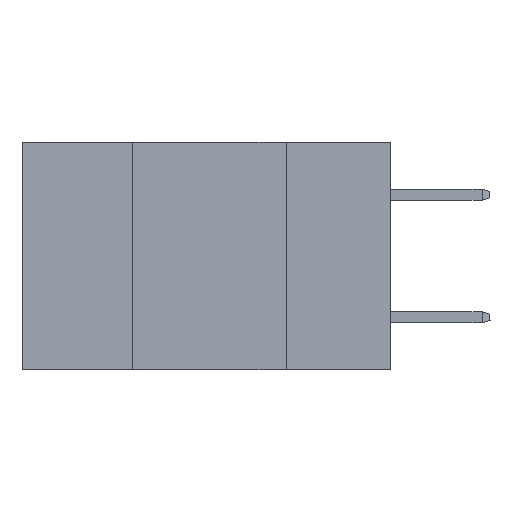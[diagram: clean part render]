
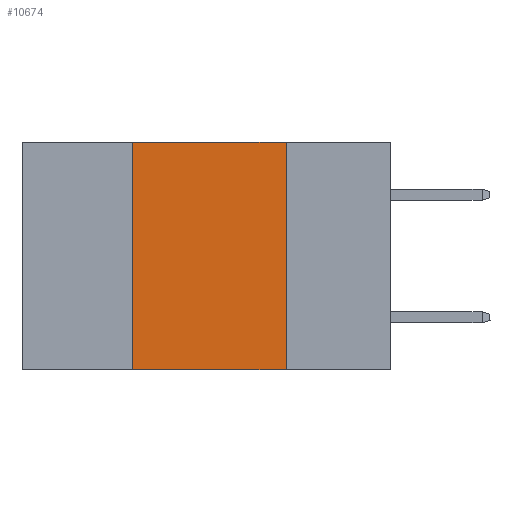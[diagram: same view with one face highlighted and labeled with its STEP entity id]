
A CAD part, left-side view. The second image highlights one B-rep face of the part: STEP entity #10674.
In plain terms, the highlighted planar face has unit normal (-1, 0, 0).
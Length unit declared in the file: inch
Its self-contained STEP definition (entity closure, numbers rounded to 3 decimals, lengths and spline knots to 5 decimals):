
#13 = PLANE ( 'NONE',  #9942 ) ;
#1749 = LINE ( 'NONE', #10028, #11382 ) ;
#1884 = VERTEX_POINT ( 'NONE', #17189 ) ;
#2172 = LINE ( 'NONE', #11243, #21198 ) ;
#3057 = LINE ( 'NONE', #11791, #22034 ) ;
#3492 = EDGE_CURVE ( 'NONE', #21601, #15595, #1749, .T. ) ;
#4226 = CARTESIAN_POINT ( 'NONE',  ( 0., 0.17, 0. ) ) ;
#4954 = VECTOR ( 'NONE', #22202, 39.37008 ) ;
#5994 = DIRECTION ( 'NONE',  ( 1., 0., 0. ) ) ;
#6545 = EDGE_CURVE ( 'NONE', #15595, #11756, #2172, .T. ) ;
#6612 = EDGE_CURVE ( 'NONE', #1884, #21601, #10068, .T. ) ;
#6679 = EDGE_CURVE ( 'NONE', #1884, #11756, #3057, .T. ) ;
#7358 = ORIENTED_EDGE ( 'NONE', *, *, #6545, .F. ) ;
#7449 = ORIENTED_EDGE ( 'NONE', *, *, #3492, .F. ) ;
#7571 = ORIENTED_EDGE ( 'NONE', *, *, #6612, .F. ) ;
#7622 = ORIENTED_EDGE ( 'NONE', *, *, #6679, .T. ) ;
#9595 = DIRECTION ( 'NONE',  ( 0., 0., -1. ) ) ;
#9681 = FACE_OUTER_BOUND ( 'NONE', #14963, .T. ) ;
#9942 = AXIS2_PLACEMENT_3D ( 'NONE', #16918, #5994, #18689 ) ;
#10028 = CARTESIAN_POINT ( 'NONE',  ( 0., 0.6, 0. ) ) ;
#10068 = LINE ( 'NONE', #11551, #4954 ) ;
#10572 = CARTESIAN_POINT ( 'NONE',  ( 0., 0.17, -0.37 ) ) ;
#10674 = ADVANCED_FACE ( 'NONE', ( #9681 ), #13, .F. ) ;
#11243 = CARTESIAN_POINT ( 'NONE',  ( 0., 0.17, 0. ) ) ;
#11382 = VECTOR ( 'NONE', #13678, 39.37008 ) ;
#11551 = CARTESIAN_POINT ( 'NONE',  ( 0., 0.42, 0. ) ) ;
#11756 = VERTEX_POINT ( 'NONE', #10572 ) ;
#11791 = CARTESIAN_POINT ( 'NONE',  ( 0., 0.6, -0.37 ) ) ;
#13630 = DIRECTION ( 'NONE',  ( 0., -1., 0. ) ) ;
#13678 = DIRECTION ( 'NONE',  ( 0., -1., 0. ) ) ;
#14963 = EDGE_LOOP ( 'NONE', ( #7358, #7449, #7571, #7622 ) ) ;
#15595 = VERTEX_POINT ( 'NONE', #4226 ) ;
#16918 = CARTESIAN_POINT ( 'NONE',  ( 0., 0.6, 0. ) ) ;
#17189 = CARTESIAN_POINT ( 'NONE',  ( 0., 0.42, -0.37 ) ) ;
#18689 = DIRECTION ( 'NONE',  ( 0., 0., -1. ) ) ;
#20741 = CARTESIAN_POINT ( 'NONE',  ( 0., 0.42, 0. ) ) ;
#21198 = VECTOR ( 'NONE', #9595, 39.37008 ) ;
#21601 = VERTEX_POINT ( 'NONE', #20741 ) ;
#22034 = VECTOR ( 'NONE', #13630, 39.37008 ) ;
#22202 = DIRECTION ( 'NONE',  ( 0., 0., 1. ) ) ;
